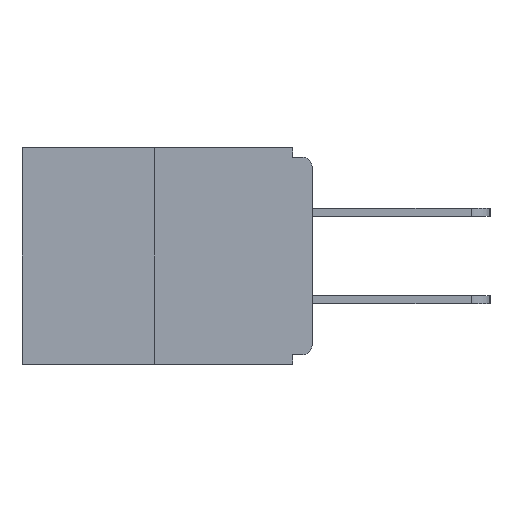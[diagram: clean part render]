
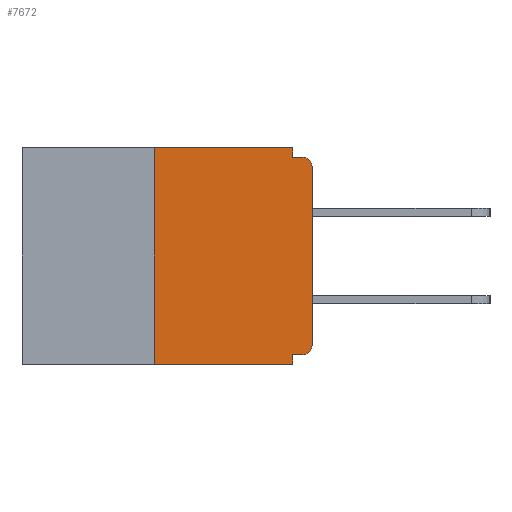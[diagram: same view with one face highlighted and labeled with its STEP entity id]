
A CAD part, left-side view. The second image highlights one B-rep face of the part: STEP entity #7672.
In plain terms, the highlighted planar face has unit normal (-1, 0, 0).
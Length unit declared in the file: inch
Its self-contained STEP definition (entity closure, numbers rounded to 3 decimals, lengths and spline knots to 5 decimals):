
#133 = VERTEX_POINT ( 'NONE', #19266 ) ;
#299 = DIRECTION ( 'NONE',  ( 0., 0., -1. ) ) ;
#573 = VERTEX_POINT ( 'NONE', #2416 ) ;
#633 = CARTESIAN_POINT ( 'NONE',  ( 0., 0.031, 0. ) ) ;
#729 = CARTESIAN_POINT ( 'NONE',  ( 0., 0.015, -0.015 ) ) ;
#1622 = CARTESIAN_POINT ( 'NONE',  ( 0., 0., 0. ) ) ;
#1696 = LINE ( 'NONE', #5311, #9413 ) ;
#1741 = VECTOR ( 'NONE', #17883, 39.37008 ) ;
#2266 = VERTEX_POINT ( 'NONE', #12649 ) ;
#2416 = CARTESIAN_POINT ( 'NONE',  ( 0., 0.031, 0. ) ) ;
#2594 = CARTESIAN_POINT ( 'NONE',  ( 0., 0., -0.328 ) ) ;
#2726 = LINE ( 'NONE', #19337, #15907 ) ;
#2777 = VECTOR ( 'NONE', #16006, 39.37008 ) ;
#2993 = ORIENTED_EDGE ( 'NONE', *, *, #18754, .T. ) ;
#3422 = EDGE_CURVE ( 'NONE', #133, #15031, #4534, .T. ) ;
#3574 = AXIS2_PLACEMENT_3D ( 'NONE', #18562, #17080, #9398 ) ;
#3707 = DIRECTION ( 'NONE',  ( 0., 0., 1. ) ) ;
#3793 = ORIENTED_EDGE ( 'NONE', *, *, #10833, .T. ) ;
#4534 = LINE ( 'NONE', #14693, #14607 ) ;
#4653 = CARTESIAN_POINT ( 'NONE',  ( 0., 0.25, 0. ) ) ;
#5249 = CIRCLE ( 'NONE', #3574, 0.015 ) ;
#5311 = CARTESIAN_POINT ( 'NONE',  ( 0., 0.25, 0. ) ) ;
#5520 = DIRECTION ( 'NONE',  ( 0., -1., 0. ) ) ;
#6272 = EDGE_CURVE ( 'NONE', #17471, #14448, #2726, .T. ) ;
#6284 = CARTESIAN_POINT ( 'NONE',  ( 0., 0.015, -0.328 ) ) ;
#6346 = CARTESIAN_POINT ( 'NONE',  ( 0., 0.031, -0.343 ) ) ;
#6385 = DIRECTION ( 'NONE',  ( 0., -1., 0. ) ) ;
#6643 = LINE ( 'NONE', #12897, #2777 ) ;
#6755 = ORIENTED_EDGE ( 'NONE', *, *, #14176, .F. ) ;
#6874 = ORIENTED_EDGE ( 'NONE', *, *, #12925, .F. ) ;
#7120 = LINE ( 'NONE', #1622, #18789 ) ;
#7291 = VERTEX_POINT ( 'NONE', #13725 ) ;
#7672 = ADVANCED_FACE ( 'NONE', ( #12769 ), #12425, .F. ) ;
#8011 = DIRECTION ( 'NONE',  ( 0., 0., 1. ) ) ;
#8094 = DIRECTION ( 'NONE',  ( -1., 0., 0. ) ) ;
#8593 = EDGE_LOOP ( 'NONE', ( #12515, #6755, #12644, #11432, #6874, #17242, #3793, #2993, #15553, #16303 ) ) ;
#9193 = EDGE_CURVE ( 'NONE', #573, #133, #10286, .T. ) ;
#9252 = CIRCLE ( 'NONE', #9863, 0.015 ) ;
#9398 = DIRECTION ( 'NONE',  ( 0., 0., -1. ) ) ;
#9413 = VECTOR ( 'NONE', #3707, 39.37008 ) ;
#9696 = CARTESIAN_POINT ( 'NONE',  ( 0., 0.015, -0.313 ) ) ;
#9863 = AXIS2_PLACEMENT_3D ( 'NONE', #9696, #8094, #17343 ) ;
#10286 = LINE ( 'NONE', #633, #10762 ) ;
#10377 = EDGE_CURVE ( 'NONE', #7291, #14448, #6643, .T. ) ;
#10762 = VECTOR ( 'NONE', #11553, 39.37008 ) ;
#10833 = EDGE_CURVE ( 'NONE', #15005, #2266, #7120, .T. ) ;
#11432 = ORIENTED_EDGE ( 'NONE', *, *, #6272, .F. ) ;
#11553 = DIRECTION ( 'NONE',  ( 0., 0., -1. ) ) ;
#12120 = VERTEX_POINT ( 'NONE', #6284 ) ;
#12425 = PLANE ( 'NONE',  #17301 ) ;
#12435 = DIRECTION ( 'NONE',  ( 0., 0., -1. ) ) ;
#12493 = CARTESIAN_POINT ( 'NONE',  ( 0., 0.46, 0. ) ) ;
#12515 = ORIENTED_EDGE ( 'NONE', *, *, #15542, .F. ) ;
#12644 = ORIENTED_EDGE ( 'NONE', *, *, #10377, .T. ) ;
#12649 = CARTESIAN_POINT ( 'NONE',  ( 0., 0., -0.03 ) ) ;
#12677 = CARTESIAN_POINT ( 'NONE',  ( 0., 0.46, 0. ) ) ;
#12769 = FACE_OUTER_BOUND ( 'NONE', #8593, .T. ) ;
#12846 = VECTOR ( 'NONE', #6385, 39.37008 ) ;
#12897 = CARTESIAN_POINT ( 'NONE',  ( 0., 0.46, -0.343 ) ) ;
#12925 = EDGE_CURVE ( 'NONE', #12120, #17471, #17507, .T. ) ;
#13725 = CARTESIAN_POINT ( 'NONE',  ( 0., 0.25, -0.343 ) ) ;
#14176 = EDGE_CURVE ( 'NONE', #7291, #18883, #1696, .T. ) ;
#14448 = VERTEX_POINT ( 'NONE', #6346 ) ;
#14607 = VECTOR ( 'NONE', #5520, 39.37008 ) ;
#14693 = CARTESIAN_POINT ( 'NONE',  ( 0., 0., -0.015 ) ) ;
#15005 = VERTEX_POINT ( 'NONE', #17156 ) ;
#15031 = VERTEX_POINT ( 'NONE', #729 ) ;
#15155 = EDGE_CURVE ( 'NONE', #12120, #15005, #9252, .T. ) ;
#15462 = LINE ( 'NONE', #12677, #12846 ) ;
#15542 = EDGE_CURVE ( 'NONE', #18883, #573, #15462, .T. ) ;
#15553 = ORIENTED_EDGE ( 'NONE', *, *, #3422, .F. ) ;
#15907 = VECTOR ( 'NONE', #12435, 39.37008 ) ;
#16006 = DIRECTION ( 'NONE',  ( 0., -1., 0. ) ) ;
#16303 = ORIENTED_EDGE ( 'NONE', *, *, #9193, .F. ) ;
#16324 = CARTESIAN_POINT ( 'NONE',  ( 0., 0.031, -0.328 ) ) ;
#17080 = DIRECTION ( 'NONE',  ( -1., 0., 0. ) ) ;
#17156 = CARTESIAN_POINT ( 'NONE',  ( 0., 0., -0.313 ) ) ;
#17188 = DIRECTION ( 'NONE',  ( 1., 0., 0. ) ) ;
#17242 = ORIENTED_EDGE ( 'NONE', *, *, #15155, .T. ) ;
#17301 = AXIS2_PLACEMENT_3D ( 'NONE', #12493, #17188, #299 ) ;
#17343 = DIRECTION ( 'NONE',  ( 0., 0., -1. ) ) ;
#17471 = VERTEX_POINT ( 'NONE', #16324 ) ;
#17507 = LINE ( 'NONE', #2594, #1741 ) ;
#17883 = DIRECTION ( 'NONE',  ( 0., 1., 0. ) ) ;
#18562 = CARTESIAN_POINT ( 'NONE',  ( 0., 0.015, -0.03 ) ) ;
#18754 = EDGE_CURVE ( 'NONE', #2266, #15031, #5249, .T. ) ;
#18789 = VECTOR ( 'NONE', #8011, 39.37008 ) ;
#18883 = VERTEX_POINT ( 'NONE', #4653 ) ;
#19266 = CARTESIAN_POINT ( 'NONE',  ( 0., 0.031, -0.015 ) ) ;
#19337 = CARTESIAN_POINT ( 'NONE',  ( 0., 0.031, -0.343 ) ) ;
